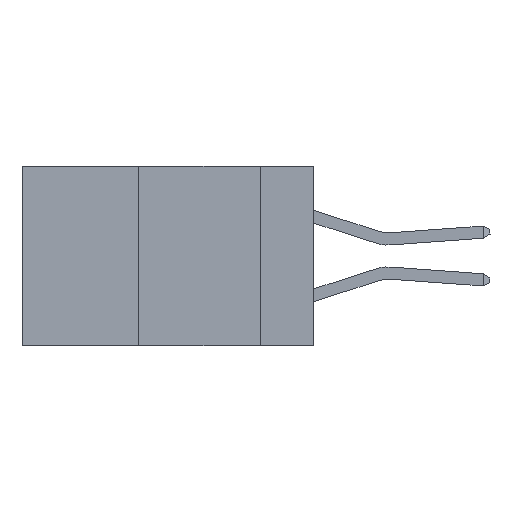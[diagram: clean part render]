
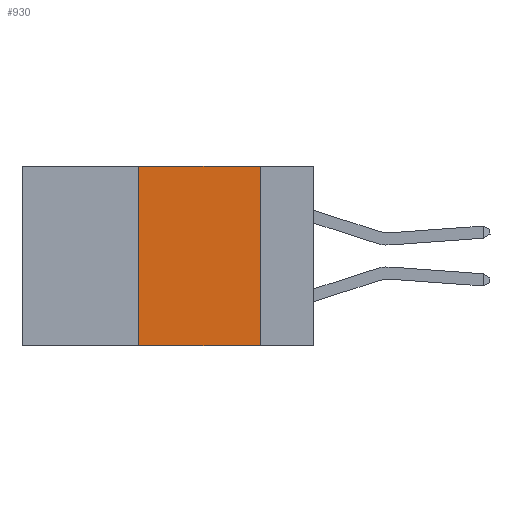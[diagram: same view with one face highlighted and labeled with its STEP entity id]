
A CAD part, left-side view. The second image highlights one B-rep face of the part: STEP entity #930.
In plain terms, the highlighted planar face has unit normal (-1, 0, 0).
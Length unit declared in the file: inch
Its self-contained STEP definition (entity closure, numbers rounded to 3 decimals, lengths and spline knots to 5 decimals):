
#930 = ADVANCED_FACE ( 'NONE', ( #2168 ), #18531, .F. ) ;
#2168 = FACE_OUTER_BOUND ( 'NONE', #17952, .T. ) ;
#4571 = LINE ( 'NONE', #14853, #8238 ) ;
#4630 = ORIENTED_EDGE ( 'NONE', *, *, #5273, .T. ) ;
#4819 = EDGE_CURVE ( 'NONE', #21815, #14370, #5020, .T. ) ;
#5020 = LINE ( 'NONE', #20644, #11231 ) ;
#5273 = EDGE_CURVE ( 'NONE', #21815, #8486, #13429, .T. ) ;
#5906 = CARTESIAN_POINT ( 'NONE',  ( 0., 0.6, -0.37 ) ) ;
#6174 = ORIENTED_EDGE ( 'NONE', *, *, #9558, .F. ) ;
#6231 = DIRECTION ( 'NONE',  ( 0., -1., 0. ) ) ;
#7405 = DIRECTION ( 'NONE',  ( 0., 0., -1. ) ) ;
#8238 = VECTOR ( 'NONE', #7405, 39.37008 ) ;
#8486 = VERTEX_POINT ( 'NONE', #20584 ) ;
#9410 = ORIENTED_EDGE ( 'NONE', *, *, #4819, .F. ) ;
#9558 = EDGE_CURVE ( 'NONE', #14370, #19444, #17281, .T. ) ;
#11231 = VECTOR ( 'NONE', #22723, 39.37008 ) ;
#11322 = DIRECTION ( 'NONE',  ( 0., 0., -1. ) ) ;
#12692 = AXIS2_PLACEMENT_3D ( 'NONE', #16574, #16500, #11322 ) ;
#13429 = LINE ( 'NONE', #5906, #18782 ) ;
#14370 = VERTEX_POINT ( 'NONE', #19227 ) ;
#14853 = CARTESIAN_POINT ( 'NONE',  ( 0., 0.11, 0. ) ) ;
#15374 = CARTESIAN_POINT ( 'NONE',  ( 0., 0.6, 0. ) ) ;
#16500 = DIRECTION ( 'NONE',  ( 1., 0., 0. ) ) ;
#16574 = CARTESIAN_POINT ( 'NONE',  ( 0., 0.6, 0. ) ) ;
#17281 = LINE ( 'NONE', #15374, #21848 ) ;
#17952 = EDGE_LOOP ( 'NONE', ( #18896, #6174, #9410, #4630 ) ) ;
#18531 = PLANE ( 'NONE',  #12692 ) ;
#18782 = VECTOR ( 'NONE', #6231, 39.37008 ) ;
#18896 = ORIENTED_EDGE ( 'NONE', *, *, #21686, .F. ) ;
#19126 = CARTESIAN_POINT ( 'NONE',  ( 0., 0.36, -0.37 ) ) ;
#19157 = DIRECTION ( 'NONE',  ( 0., -1., 0. ) ) ;
#19227 = CARTESIAN_POINT ( 'NONE',  ( 0., 0.36, 0. ) ) ;
#19444 = VERTEX_POINT ( 'NONE', #20869 ) ;
#20584 = CARTESIAN_POINT ( 'NONE',  ( 0., 0.11, -0.37 ) ) ;
#20644 = CARTESIAN_POINT ( 'NONE',  ( 0., 0.36, 0. ) ) ;
#20869 = CARTESIAN_POINT ( 'NONE',  ( 0., 0.11, 0. ) ) ;
#21686 = EDGE_CURVE ( 'NONE', #19444, #8486, #4571, .T. ) ;
#21815 = VERTEX_POINT ( 'NONE', #19126 ) ;
#21848 = VECTOR ( 'NONE', #19157, 39.37008 ) ;
#22723 = DIRECTION ( 'NONE',  ( 0., 0., 1. ) ) ;
